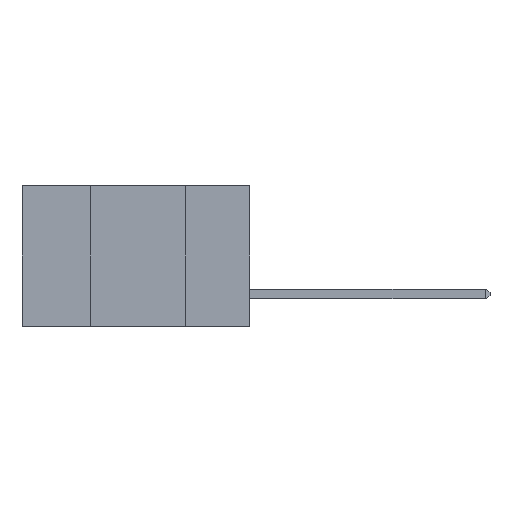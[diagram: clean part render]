
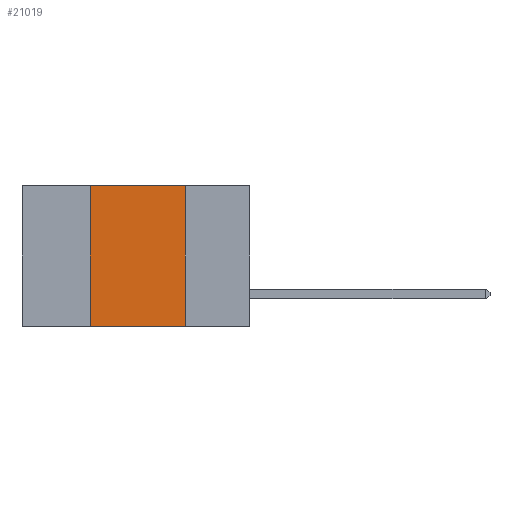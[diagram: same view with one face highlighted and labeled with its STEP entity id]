
A CAD part, left-side view. The second image highlights one B-rep face of the part: STEP entity #21019.
In plain terms, the highlighted planar face has unit normal (-1, 0, 0).
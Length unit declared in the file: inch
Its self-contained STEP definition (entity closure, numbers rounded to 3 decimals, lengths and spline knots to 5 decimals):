
#332 = EDGE_CURVE ( 'NONE', #13597, #11142, #8966, .T. ) ;
#1042 = EDGE_CURVE ( 'NONE', #11904, #11142, #2886, .T. ) ;
#1096 = CARTESIAN_POINT ( 'NONE',  ( 0., 0.6, -0.37 ) ) ;
#1745 = LINE ( 'NONE', #7488, #20089 ) ;
#1940 = CARTESIAN_POINT ( 'NONE',  ( 0., 0.17, -0.37 ) ) ;
#2010 = CARTESIAN_POINT ( 'NONE',  ( 0., 0.42, 0. ) ) ;
#2294 = EDGE_LOOP ( 'NONE', ( #8364, #13731, #23374, #4623 ) ) ;
#2886 = LINE ( 'NONE', #18378, #7867 ) ;
#4623 = ORIENTED_EDGE ( 'NONE', *, *, #332, .T. ) ;
#4732 = VECTOR ( 'NONE', #20452, 39.37008 ) ;
#6455 = DIRECTION ( 'NONE',  ( 1., 0., 0. ) ) ;
#7488 = CARTESIAN_POINT ( 'NONE',  ( 0., 0.42, 0. ) ) ;
#7848 = VECTOR ( 'NONE', #17905, 39.37008 ) ;
#7867 = VECTOR ( 'NONE', #8450, 39.37008 ) ;
#8364 = ORIENTED_EDGE ( 'NONE', *, *, #1042, .F. ) ;
#8450 = DIRECTION ( 'NONE',  ( 0., 0., -1. ) ) ;
#8966 = LINE ( 'NONE', #1096, #7848 ) ;
#9865 = FACE_OUTER_BOUND ( 'NONE', #2294, .T. ) ;
#10092 = CARTESIAN_POINT ( 'NONE',  ( 0., 0.42, -0.37 ) ) ;
#11142 = VERTEX_POINT ( 'NONE', #1940 ) ;
#11831 = CARTESIAN_POINT ( 'NONE',  ( 0., 0.6, 0. ) ) ;
#11904 = VERTEX_POINT ( 'NONE', #20550 ) ;
#13597 = VERTEX_POINT ( 'NONE', #10092 ) ;
#13731 = ORIENTED_EDGE ( 'NONE', *, *, #20830, .F. ) ;
#17341 = PLANE ( 'NONE',  #21896 ) ;
#17905 = DIRECTION ( 'NONE',  ( 0., -1., 0. ) ) ;
#18378 = CARTESIAN_POINT ( 'NONE',  ( 0., 0.17, 0. ) ) ;
#19161 = DIRECTION ( 'NONE',  ( 0., 0., -1. ) ) ;
#20089 = VECTOR ( 'NONE', #22083, 39.37008 ) ;
#20452 = DIRECTION ( 'NONE',  ( 0., -1., 0. ) ) ;
#20550 = CARTESIAN_POINT ( 'NONE',  ( 0., 0.17, 0. ) ) ;
#20830 = EDGE_CURVE ( 'NONE', #22197, #11904, #23486, .T. ) ;
#21019 = ADVANCED_FACE ( 'NONE', ( #9865 ), #17341, .F. ) ;
#21385 = EDGE_CURVE ( 'NONE', #13597, #22197, #1745, .T. ) ;
#21896 = AXIS2_PLACEMENT_3D ( 'NONE', #11831, #6455, #19161 ) ;
#22083 = DIRECTION ( 'NONE',  ( 0., 0., 1. ) ) ;
#22197 = VERTEX_POINT ( 'NONE', #2010 ) ;
#22266 = CARTESIAN_POINT ( 'NONE',  ( 0., 0.6, 0. ) ) ;
#23374 = ORIENTED_EDGE ( 'NONE', *, *, #21385, .F. ) ;
#23486 = LINE ( 'NONE', #22266, #4732 ) ;
